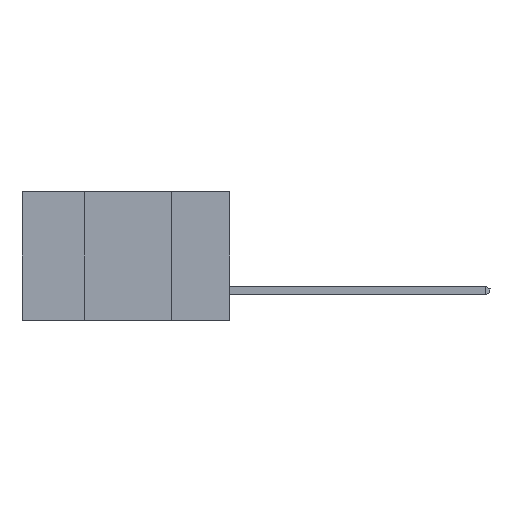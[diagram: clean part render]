
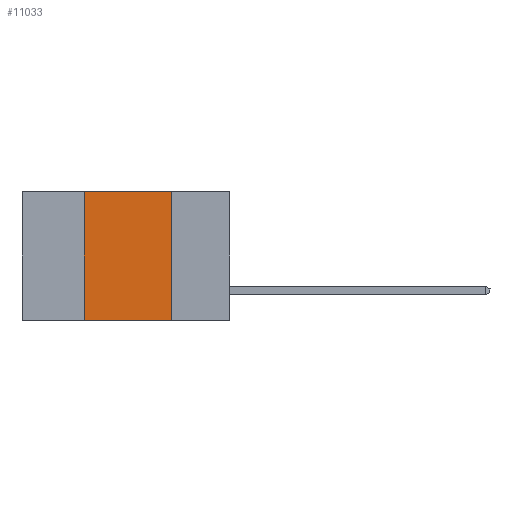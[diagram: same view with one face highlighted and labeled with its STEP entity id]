
A CAD part, left-side view. The second image highlights one B-rep face of the part: STEP entity #11033.
In plain terms, the highlighted planar face has unit normal (-1, 0, 0).
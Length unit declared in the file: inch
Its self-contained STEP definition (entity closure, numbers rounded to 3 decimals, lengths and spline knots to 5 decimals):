
#1541 = DIRECTION ( 'NONE',  ( 1., 0., 0. ) ) ;
#1547 = ORIENTED_EDGE ( 'NONE', *, *, #18329, .F. ) ;
#2040 = CARTESIAN_POINT ( 'NONE',  ( 0., 0.6, -0.37 ) ) ;
#3094 = CARTESIAN_POINT ( 'NONE',  ( 0., 0.42, -0.37 ) ) ;
#4749 = LINE ( 'NONE', #3094, #16631 ) ;
#4874 = CARTESIAN_POINT ( 'NONE',  ( 0., 0.17, -0.37 ) ) ;
#4909 = VECTOR ( 'NONE', #14859, 39.37008 ) ;
#5259 = ORIENTED_EDGE ( 'NONE', *, *, #16232, .T. ) ;
#5808 = CARTESIAN_POINT ( 'NONE',  ( 0., 0.17, -0.37 ) ) ;
#7351 = EDGE_CURVE ( 'NONE', #9703, #13309, #4749, .T. ) ;
#8532 = CARTESIAN_POINT ( 'NONE',  ( 0., 0.6, 0. ) ) ;
#8618 = LINE ( 'NONE', #2040, #13557 ) ;
#9337 = DIRECTION ( 'NONE',  ( 0., 0., 1. ) ) ;
#9667 = LINE ( 'NONE', #4874, #15937 ) ;
#9703 = VERTEX_POINT ( 'NONE', #13700 ) ;
#10187 = LINE ( 'NONE', #8532, #4909 ) ;
#10705 = VERTEX_POINT ( 'NONE', #15627 ) ;
#10728 = DIRECTION ( 'NONE',  ( 0., 0., -1. ) ) ;
#11033 = ADVANCED_FACE ( 'NONE', ( #12578 ), #15499, .F. ) ;
#11576 = EDGE_LOOP ( 'NONE', ( #1547, #14669, #19886, #5259 ) ) ;
#12578 = FACE_OUTER_BOUND ( 'NONE', #11576, .T. ) ;
#13083 = CARTESIAN_POINT ( 'NONE',  ( 0., 0.42, 0. ) ) ;
#13309 = VERTEX_POINT ( 'NONE', #13083 ) ;
#13557 = VECTOR ( 'NONE', #19800, 39.37008 ) ;
#13700 = CARTESIAN_POINT ( 'NONE',  ( 0., 0.42, -0.37 ) ) ;
#14669 = ORIENTED_EDGE ( 'NONE', *, *, #15881, .F. ) ;
#14859 = DIRECTION ( 'NONE',  ( 0., -1., 0. ) ) ;
#15499 = PLANE ( 'NONE',  #18112 ) ;
#15627 = CARTESIAN_POINT ( 'NONE',  ( 0., 0.17, 0. ) ) ;
#15881 = EDGE_CURVE ( 'NONE', #13309, #10705, #10187, .T. ) ;
#15937 = VECTOR ( 'NONE', #16109, 39.37008 ) ;
#16109 = DIRECTION ( 'NONE',  ( 0., 0., -1. ) ) ;
#16232 = EDGE_CURVE ( 'NONE', #9703, #17269, #8618, .T. ) ;
#16631 = VECTOR ( 'NONE', #9337, 39.37008 ) ;
#17269 = VERTEX_POINT ( 'NONE', #5808 ) ;
#18112 = AXIS2_PLACEMENT_3D ( 'NONE', #18813, #1541, #10728 ) ;
#18329 = EDGE_CURVE ( 'NONE', #10705, #17269, #9667, .T. ) ;
#18813 = CARTESIAN_POINT ( 'NONE',  ( 0., 0.6, 0. ) ) ;
#19800 = DIRECTION ( 'NONE',  ( 0., -1., 0. ) ) ;
#19886 = ORIENTED_EDGE ( 'NONE', *, *, #7351, .F. ) ;
